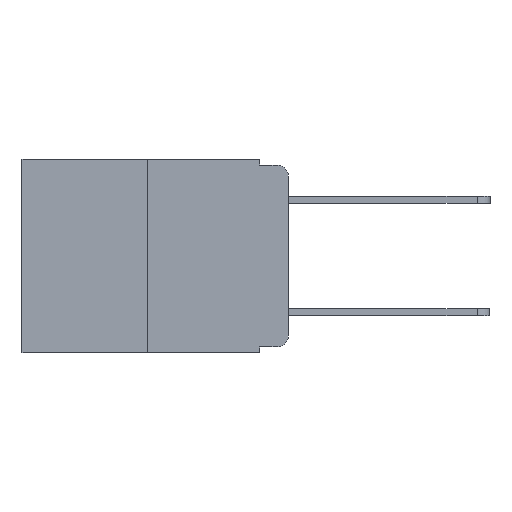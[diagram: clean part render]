
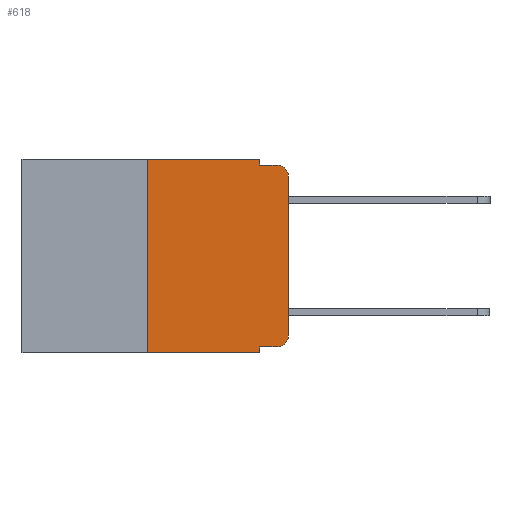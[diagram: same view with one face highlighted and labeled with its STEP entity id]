
A CAD part, left-side view. The second image highlights one B-rep face of the part: STEP entity #618.
In plain terms, the highlighted planar face has unit normal (-1, 0, 0).
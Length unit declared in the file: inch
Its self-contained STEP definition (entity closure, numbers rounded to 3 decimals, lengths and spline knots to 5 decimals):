
#60 = CARTESIAN_POINT ( 'NONE',  ( 0., 0.02, -0.313 ) ) ;
#70 = CARTESIAN_POINT ( 'NONE',  ( 0., 0.25, -0.343 ) ) ;
#420 = DIRECTION ( 'NONE',  ( 0., 0., -1. ) ) ;
#501 = CARTESIAN_POINT ( 'NONE',  ( 0., 0.02, -0.03 ) ) ;
#521 = CARTESIAN_POINT ( 'NONE',  ( 0., 0.051, -0.333 ) ) ;
#545 = EDGE_CURVE ( 'NONE', #1002, #5186, #3622, .T. ) ;
#618 = ADVANCED_FACE ( 'NONE', ( #2991 ), #8883, .F. ) ;
#694 = VECTOR ( 'NONE', #3703, 39.37008 ) ;
#755 = VERTEX_POINT ( 'NONE', #521 ) ;
#1002 = VERTEX_POINT ( 'NONE', #1113 ) ;
#1078 = DIRECTION ( 'NONE',  ( 0., 0., -1. ) ) ;
#1113 = CARTESIAN_POINT ( 'NONE',  ( 0., 0.051, -0.01 ) ) ;
#1542 = DIRECTION ( 'NONE',  ( 0., 0., -1. ) ) ;
#1569 = VECTOR ( 'NONE', #10554, 39.37008 ) ;
#1684 = VERTEX_POINT ( 'NONE', #9103 ) ;
#1688 = VECTOR ( 'NONE', #2529, 39.37008 ) ;
#2404 = EDGE_CURVE ( 'NONE', #2688, #2902, #8393, .T. ) ;
#2529 = DIRECTION ( 'NONE',  ( 0., 0., 1. ) ) ;
#2537 = LINE ( 'NONE', #6631, #7348 ) ;
#2613 = DIRECTION ( 'NONE',  ( 1., 0., 0. ) ) ;
#2688 = VERTEX_POINT ( 'NONE', #4207 ) ;
#2699 = CARTESIAN_POINT ( 'NONE',  ( 0., 0.473, 0. ) ) ;
#2734 = DIRECTION ( 'NONE',  ( 0., -1., 0. ) ) ;
#2902 = VERTEX_POINT ( 'NONE', #11903 ) ;
#2991 = FACE_OUTER_BOUND ( 'NONE', #11466, .T. ) ;
#3251 = AXIS2_PLACEMENT_3D ( 'NONE', #501, #7335, #1542 ) ;
#3308 = VECTOR ( 'NONE', #4821, 39.37008 ) ;
#3466 = CARTESIAN_POINT ( 'NONE',  ( 0., 0., -0.313 ) ) ;
#3545 = CARTESIAN_POINT ( 'NONE',  ( 0., 0.25, 0. ) ) ;
#3622 = LINE ( 'NONE', #8159, #3308 ) ;
#3703 = DIRECTION ( 'NONE',  ( 0., -1., 0. ) ) ;
#3911 = CARTESIAN_POINT ( 'NONE',  ( 0., 0., 0. ) ) ;
#4207 = CARTESIAN_POINT ( 'NONE',  ( 0., 0.25, 0. ) ) ;
#4611 = ORIENTED_EDGE ( 'NONE', *, *, #9992, .T. ) ;
#4701 = CARTESIAN_POINT ( 'NONE',  ( 0., 0.02, -0.333 ) ) ;
#4747 = VERTEX_POINT ( 'NONE', #3466 ) ;
#4821 = DIRECTION ( 'NONE',  ( 0., -1., 0. ) ) ;
#4936 = ORIENTED_EDGE ( 'NONE', *, *, #545, .F. ) ;
#4951 = VERTEX_POINT ( 'NONE', #4701 ) ;
#5186 = VERTEX_POINT ( 'NONE', #8452 ) ;
#5253 = CARTESIAN_POINT ( 'NONE',  ( 0., 0.051, -0.333 ) ) ;
#5264 = CARTESIAN_POINT ( 'NONE',  ( 0., 0., -0.03 ) ) ;
#5462 = VECTOR ( 'NONE', #6212, 39.37008 ) ;
#5487 = EDGE_CURVE ( 'NONE', #755, #1684, #11839, .T. ) ;
#5673 = AXIS2_PLACEMENT_3D ( 'NONE', #11173, #2613, #420 ) ;
#5829 = CIRCLE ( 'NONE', #3251, 0.02 ) ;
#5898 = ORIENTED_EDGE ( 'NONE', *, *, #2404, .F. ) ;
#6212 = DIRECTION ( 'NONE',  ( 0., -1., 0. ) ) ;
#6531 = LINE ( 'NONE', #8408, #8930 ) ;
#6631 = CARTESIAN_POINT ( 'NONE',  ( 0., 0.051, 0. ) ) ;
#6801 = CIRCLE ( 'NONE', #11291, 0.02 ) ;
#6871 = LINE ( 'NONE', #3545, #1688 ) ;
#6940 = DIRECTION ( 'NONE',  ( -1., 0., 0. ) ) ;
#7166 = ORIENTED_EDGE ( 'NONE', *, *, #9351, .T. ) ;
#7335 = DIRECTION ( 'NONE',  ( -1., 0., 0. ) ) ;
#7348 = VECTOR ( 'NONE', #7550, 39.37008 ) ;
#7453 = ORIENTED_EDGE ( 'NONE', *, *, #10963, .F. ) ;
#7550 = DIRECTION ( 'NONE',  ( 0., 0., -1. ) ) ;
#7783 = ORIENTED_EDGE ( 'NONE', *, *, #11801, .T. ) ;
#7804 = VERTEX_POINT ( 'NONE', #5264 ) ;
#7954 = EDGE_CURVE ( 'NONE', #11179, #2688, #6871, .T. ) ;
#8159 = CARTESIAN_POINT ( 'NONE',  ( 0., 0.051, -0.01 ) ) ;
#8393 = LINE ( 'NONE', #2699, #694 ) ;
#8408 = CARTESIAN_POINT ( 'NONE',  ( 0., 0.473, -0.343 ) ) ;
#8452 = CARTESIAN_POINT ( 'NONE',  ( 0., 0.02, -0.01 ) ) ;
#8883 = PLANE ( 'NONE',  #5673 ) ;
#8897 = LINE ( 'NONE', #3911, #11023 ) ;
#8930 = VECTOR ( 'NONE', #2734, 39.37008 ) ;
#9103 = CARTESIAN_POINT ( 'NONE',  ( 0., 0.051, -0.343 ) ) ;
#9250 = EDGE_CURVE ( 'NONE', #7804, #5186, #5829, .T. ) ;
#9351 = EDGE_CURVE ( 'NONE', #11179, #1684, #6531, .T. ) ;
#9449 = ORIENTED_EDGE ( 'NONE', *, *, #5487, .F. ) ;
#9666 = CARTESIAN_POINT ( 'NONE',  ( 0., 0.051, 0. ) ) ;
#9790 = ORIENTED_EDGE ( 'NONE', *, *, #11064, .T. ) ;
#9992 = EDGE_CURVE ( 'NONE', #4951, #4747, #6801, .T. ) ;
#10304 = LINE ( 'NONE', #5253, #5462 ) ;
#10378 = DIRECTION ( 'NONE',  ( 0., 0., 1. ) ) ;
#10554 = DIRECTION ( 'NONE',  ( 0., 0., -1. ) ) ;
#10837 = ORIENTED_EDGE ( 'NONE', *, *, #7954, .F. ) ;
#10963 = EDGE_CURVE ( 'NONE', #2902, #1002, #2537, .T. ) ;
#11023 = VECTOR ( 'NONE', #10378, 39.37008 ) ;
#11064 = EDGE_CURVE ( 'NONE', #4747, #7804, #8897, .T. ) ;
#11173 = CARTESIAN_POINT ( 'NONE',  ( 0., 0.473, 0. ) ) ;
#11179 = VERTEX_POINT ( 'NONE', #70 ) ;
#11291 = AXIS2_PLACEMENT_3D ( 'NONE', #60, #6940, #1078 ) ;
#11466 = EDGE_LOOP ( 'NONE', ( #9790, #11644, #4936, #7453, #5898, #10837, #7166, #9449, #7783, #4611 ) ) ;
#11644 = ORIENTED_EDGE ( 'NONE', *, *, #9250, .T. ) ;
#11801 = EDGE_CURVE ( 'NONE', #755, #4951, #10304, .T. ) ;
#11839 = LINE ( 'NONE', #9666, #1569 ) ;
#11903 = CARTESIAN_POINT ( 'NONE',  ( 0., 0.051, 0. ) ) ;
